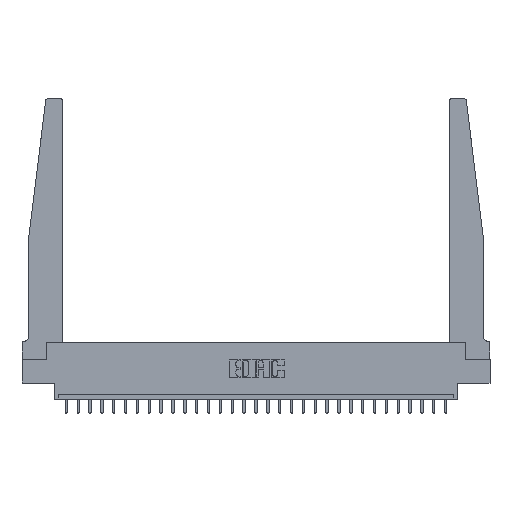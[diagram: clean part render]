
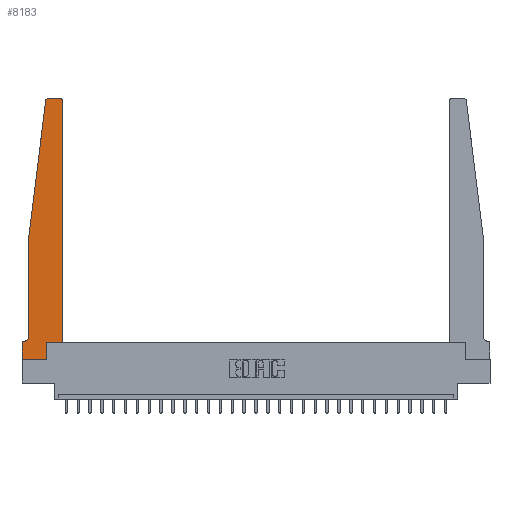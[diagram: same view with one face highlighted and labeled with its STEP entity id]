
A CAD part, top view. The second image highlights one B-rep face of the part: STEP entity #8183.
In plain terms, the highlighted planar face has unit normal (0, 0, 1).
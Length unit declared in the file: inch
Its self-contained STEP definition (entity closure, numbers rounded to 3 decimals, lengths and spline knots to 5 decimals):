
#97 = ORIENTED_EDGE ( 'NONE', *, *, #26168, .T. ) ;
#145 = DIRECTION ( 'NONE',  ( 1., 0., 0. ) ) ;
#346 = LINE ( 'NONE', #25979, #7757 ) ;
#507 = FACE_OUTER_BOUND ( 'NONE', #12500, .T. ) ;
#682 = CARTESIAN_POINT ( 'NONE',  ( 0.2605, 0.18, 0.37 ) ) ;
#905 = LINE ( 'NONE', #3511, #24353 ) ;
#1135 = DIRECTION ( 'NONE',  ( 0., 0., -1. ) ) ;
#1565 = LINE ( 'NONE', #10106, #17379 ) ;
#1774 = VECTOR ( 'NONE', #2226, 39.37008 ) ;
#1918 = AXIS2_PLACEMENT_3D ( 'NONE', #4683, #4860, #6633 ) ;
#2076 = VERTEX_POINT ( 'NONE', #7642 ) ;
#2191 = CARTESIAN_POINT ( 'NONE',  ( 0.2605, 0., 0.37 ) ) ;
#2226 = DIRECTION ( 'NONE',  ( -1., 0., 0. ) ) ;
#2411 = ORIENTED_EDGE ( 'NONE', *, *, #20979, .T. ) ;
#3039 = CARTESIAN_POINT ( 'NONE',  ( 0.015, 0.2375, 0.37 ) ) ;
#3103 = CARTESIAN_POINT ( 'NONE',  ( 0.24675, 2.72367, 0.37 ) ) ;
#3206 = CARTESIAN_POINT ( 'NONE',  ( 0., 0., 0.37 ) ) ;
#3511 = CARTESIAN_POINT ( 'NONE',  ( 0., 0., 0.37 ) ) ;
#3597 = ORIENTED_EDGE ( 'NONE', *, *, #8484, .T. ) ;
#3888 = PLANE ( 'NONE',  #25668 ) ;
#4039 = ORIENTED_EDGE ( 'NONE', *, *, #21826, .T. ) ;
#4683 = CARTESIAN_POINT ( 'NONE',  ( 0.395, 2.72, 0.37 ) ) ;
#4860 = DIRECTION ( 'NONE',  ( 0., 0., 1. ) ) ;
#5165 = VERTEX_POINT ( 'NONE', #2191 ) ;
#5255 = DIRECTION ( 'NONE',  ( 0., -1., 0. ) ) ;
#5305 = LINE ( 'NONE', #24755, #1774 ) ;
#5638 = EDGE_CURVE ( 'NONE', #5165, #19823, #6050, .T. ) ;
#5742 = VECTOR ( 'NONE', #8485, 39.37008 ) ;
#6050 = LINE ( 'NONE', #20597, #26613 ) ;
#6633 = DIRECTION ( 'NONE',  ( 1., 0., 0. ) ) ;
#6634 = DIRECTION ( 'NONE',  ( -1., 0., 0. ) ) ;
#6810 = CARTESIAN_POINT ( 'NONE',  ( 0.065, 0.1875, 0.37 ) ) ;
#6928 = VERTEX_POINT ( 'NONE', #7527 ) ;
#7515 = DIRECTION ( 'NONE',  ( -1., 0., 0. ) ) ;
#7527 = CARTESIAN_POINT ( 'NONE',  ( 0.425, 2.72, 0.37 ) ) ;
#7642 = CARTESIAN_POINT ( 'NONE',  ( 0., 0.1875, 0.37 ) ) ;
#7747 = VERTEX_POINT ( 'NONE', #22839 ) ;
#7757 = VECTOR ( 'NONE', #25804, 39.37008 ) ;
#8146 = VERTEX_POINT ( 'NONE', #17603 ) ;
#8183 = ADVANCED_FACE ( 'NONE', ( #507 ), #3888, .T. ) ;
#8257 = VECTOR ( 'NONE', #145, 39.37008 ) ;
#8484 = EDGE_CURVE ( 'NONE', #6928, #7747, #17936, .T. ) ;
#8485 = DIRECTION ( 'NONE',  ( 0., -1., 0. ) ) ;
#8573 = CARTESIAN_POINT ( 'NONE',  ( 0.065, 1.25, 0.37 ) ) ;
#9747 = CIRCLE ( 'NONE', #22258, 0.03 ) ;
#10106 = CARTESIAN_POINT ( 'NONE',  ( 0.065, 1.25, 0.37 ) ) ;
#11254 = ORIENTED_EDGE ( 'NONE', *, *, #19238, .T. ) ;
#11257 = ORIENTED_EDGE ( 'NONE', *, *, #13438, .T. ) ;
#11812 = LINE ( 'NONE', #3206, #13437 ) ;
#12065 = DIRECTION ( 'NONE',  ( 0., 0., 1. ) ) ;
#12500 = EDGE_LOOP ( 'NONE', ( #2411, #4039, #13534, #11257, #20411, #11254, #97, #14623, #19878, #24069, #23147, #3597 ) ) ;
#12743 = CARTESIAN_POINT ( 'NONE',  ( 0.065, 1.25, 0.37 ) ) ;
#13437 = VECTOR ( 'NONE', #5255, 39.37008 ) ;
#13438 = EDGE_CURVE ( 'NONE', #25487, #18343, #24409, .T. ) ;
#13534 = ORIENTED_EDGE ( 'NONE', *, *, #18312, .T. ) ;
#14340 = EDGE_CURVE ( 'NONE', #24557, #5165, #905, .T. ) ;
#14623 = ORIENTED_EDGE ( 'NONE', *, *, #14340, .T. ) ;
#14930 = EDGE_CURVE ( 'NONE', #19823, #8146, #23056, .T. ) ;
#15994 = DIRECTION ( 'NONE',  ( -0.122, -0.992, 0. ) ) ;
#16024 = CIRCLE ( 'NONE', #16607, 0.05 ) ;
#16237 = DIRECTION ( 'NONE',  ( 1., 0., 0. ) ) ;
#16244 = DIRECTION ( 'NONE',  ( 0., 1., 0. ) ) ;
#16321 = CARTESIAN_POINT ( 'NONE',  ( 0., 0.1875, 0.37 ) ) ;
#16607 = AXIS2_PLACEMENT_3D ( 'NONE', #3039, #1135, #7515 ) ;
#17379 = VECTOR ( 'NONE', #15994, 39.37008 ) ;
#17525 = VERTEX_POINT ( 'NONE', #3103 ) ;
#17603 = CARTESIAN_POINT ( 'NONE',  ( 0.425, 0.18, 0.37 ) ) ;
#17936 = CIRCLE ( 'NONE', #1918, 0.03 ) ;
#18312 = EDGE_CURVE ( 'NONE', #17525, #25487, #1565, .T. ) ;
#18343 = VERTEX_POINT ( 'NONE', #20107 ) ;
#18649 = CARTESIAN_POINT ( 'NONE',  ( 0.27653, 2.72, 0.37 ) ) ;
#18740 = DIRECTION ( 'NONE',  ( 0., 0., 1. ) ) ;
#19238 = EDGE_CURVE ( 'NONE', #21444, #2076, #19845, .T. ) ;
#19628 = CARTESIAN_POINT ( 'NONE',  ( 0., 0., 0.37 ) ) ;
#19823 = VERTEX_POINT ( 'NONE', #682 ) ;
#19845 = LINE ( 'NONE', #6810, #23672 ) ;
#19878 = ORIENTED_EDGE ( 'NONE', *, *, #5638, .T. ) ;
#19897 = EDGE_CURVE ( 'NONE', #18343, #21444, #16024, .T. ) ;
#20107 = CARTESIAN_POINT ( 'NONE',  ( 0.065, 0.2375, 0.37 ) ) ;
#20411 = ORIENTED_EDGE ( 'NONE', *, *, #19897, .T. ) ;
#20597 = CARTESIAN_POINT ( 'NONE',  ( 0.2605, 0.18, 0.37 ) ) ;
#20979 = EDGE_CURVE ( 'NONE', #7747, #22145, #5305, .T. ) ;
#21444 = VERTEX_POINT ( 'NONE', #24895 ) ;
#21826 = EDGE_CURVE ( 'NONE', #22145, #17525, #9747, .T. ) ;
#22145 = VERTEX_POINT ( 'NONE', #25498 ) ;
#22258 = AXIS2_PLACEMENT_3D ( 'NONE', #18649, #18740, #22721 ) ;
#22721 = DIRECTION ( 'NONE',  ( 1., 0., 0. ) ) ;
#22839 = CARTESIAN_POINT ( 'NONE',  ( 0.395, 2.75, 0.37 ) ) ;
#23056 = LINE ( 'NONE', #25041, #8257 ) ;
#23147 = ORIENTED_EDGE ( 'NONE', *, *, #24015, .T. ) ;
#23672 = VECTOR ( 'NONE', #6634, 39.37008 ) ;
#23962 = DIRECTION ( 'NONE',  ( 1., 0., 0. ) ) ;
#24015 = EDGE_CURVE ( 'NONE', #8146, #6928, #346, .T. ) ;
#24069 = ORIENTED_EDGE ( 'NONE', *, *, #14930, .T. ) ;
#24353 = VECTOR ( 'NONE', #23962, 39.37008 ) ;
#24409 = LINE ( 'NONE', #8573, #5742 ) ;
#24557 = VERTEX_POINT ( 'NONE', #19628 ) ;
#24755 = CARTESIAN_POINT ( 'NONE',  ( 0.25, 2.75, 0.37 ) ) ;
#24895 = CARTESIAN_POINT ( 'NONE',  ( 0.015, 0.1875, 0.37 ) ) ;
#25041 = CARTESIAN_POINT ( 'NONE',  ( 0.425, 0.18, 0.37 ) ) ;
#25487 = VERTEX_POINT ( 'NONE', #12743 ) ;
#25498 = CARTESIAN_POINT ( 'NONE',  ( 0.27653, 2.75, 0.37 ) ) ;
#25668 = AXIS2_PLACEMENT_3D ( 'NONE', #16321, #12065, #16237 ) ;
#25804 = DIRECTION ( 'NONE',  ( 0., 1., 0. ) ) ;
#25979 = CARTESIAN_POINT ( 'NONE',  ( 0.425, 0.18, 0.37 ) ) ;
#26168 = EDGE_CURVE ( 'NONE', #2076, #24557, #11812, .T. ) ;
#26613 = VECTOR ( 'NONE', #16244, 39.37008 ) ;
